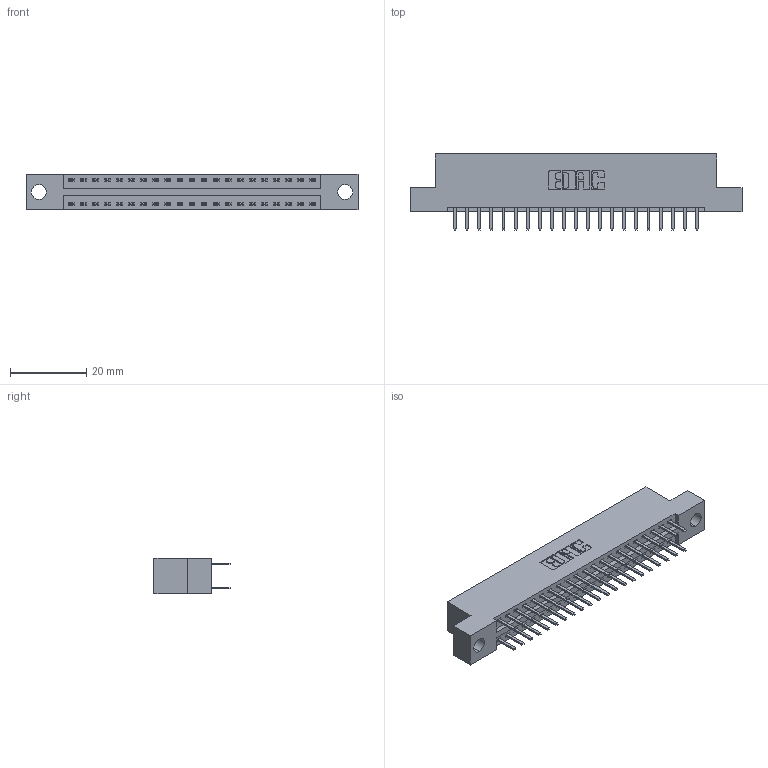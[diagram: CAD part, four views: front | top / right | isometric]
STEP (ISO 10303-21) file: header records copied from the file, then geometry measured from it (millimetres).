
FILE_DESCRIPTION (( 'STEP AP203' ), '1' );
FILE_NAME ('396-042-520-204.STEP', '2018-09-06T23:20:54', ( '' ), ( '' ), 'SwSTEP 2.0', 'SolidWorks 2016', '' );
FILE_SCHEMA (( 'CONFIG_CONTROL_DESIGN' ));
Length unit declared in the file: inch
Products named in the file (3): 346 Part_Flush Mounting Lugs - 0.156 Dia-TH; 345-292-001_345-293-120; 396-042-520-204
Assembly tree (43 placements, depth 2):
  396-042-520-204
    346 Part_Flush Mounting Lugs - 0.156 Dia-TH
    345-292-001_345-293-120  x42
Bounding box: 87.25 x 20.02 x 9.4 mm (x, y, z)
Volume: 8238.4 mm3; surface area: 10764.3 mm2
Topology: 43 solids, 43 shells, 2474 faces, 7175 edges, 4670 vertices
Faces by surface type: plane 1630, cylinder 844
Entity records: 16649 total; most frequent: CARTESIAN_POINT 2784, ORIENTED_EDGE 2706, DIRECTION 2493, EDGE_CURVE 1353, VECTOR 1133, LINE 1133, VERTEX_POINT 898, AXIS2_PLACEMENT_3D 680
